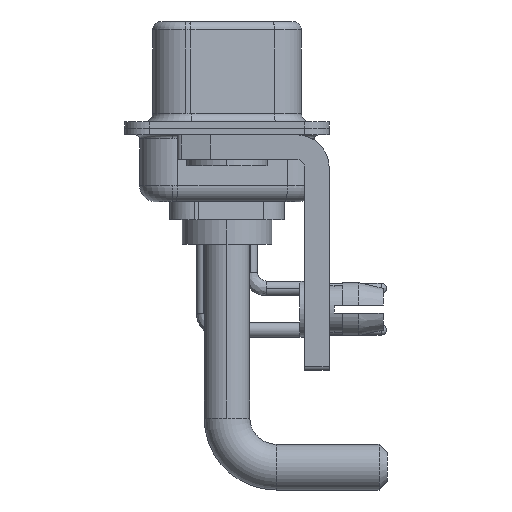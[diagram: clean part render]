
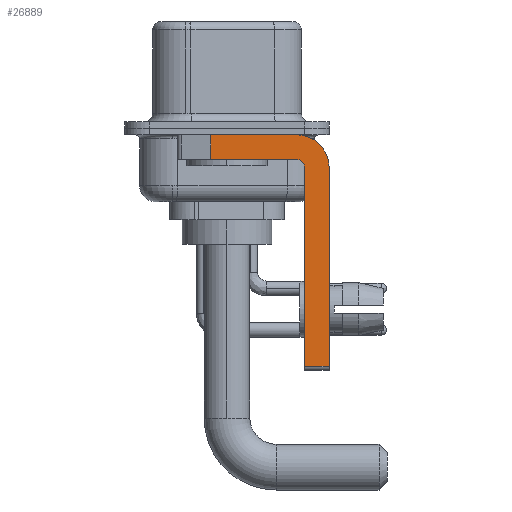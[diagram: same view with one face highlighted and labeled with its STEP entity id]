
A CAD part, left-side view. The second image highlights one B-rep face of the part: STEP entity #26889.
In plain terms, the highlighted planar face has unit normal (-1, 0, 0).
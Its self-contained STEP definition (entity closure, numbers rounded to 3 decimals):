
#29 = VERTEX_POINT ( 'NONE', #8111 ) ;
#87 = DIRECTION ( 'NONE',  ( 0., 0., 1. ) ) ;
#91 = VERTEX_POINT ( 'NONE', #766 ) ;
#352 = VECTOR ( 'NONE', #25271, 1000. ) ;
#766 = CARTESIAN_POINT ( 'NONE',  ( -2.9, 0.978, -1.9 ) ) ;
#917 = VERTEX_POINT ( 'NONE', #10196 ) ;
#934 = EDGE_LOOP ( 'NONE', ( #25266, #8101, #20002, #5341, #11977, #13872, #5453, #2150 ) ) ;
#1042 = EDGE_CURVE ( 'NONE', #917, #29, #13442, .T. ) ;
#2150 = ORIENTED_EDGE ( 'NONE', *, *, #5761, .F. ) ;
#2473 = LINE ( 'NONE', #17156, #7376 ) ;
#2628 = VECTOR ( 'NONE', #23406, 1000. ) ;
#2943 = DIRECTION ( 'NONE',  ( 0., 0., -1. ) ) ;
#3097 = EDGE_CURVE ( 'NONE', #5875, #26290, #18706, .T. ) ;
#3352 = PLANE ( 'NONE',  #24534 ) ;
#3684 = CIRCLE ( 'NONE', #23646, 2. ) ;
#4737 = CARTESIAN_POINT ( 'NONE',  ( -2.9, 0.978, -1.9 ) ) ;
#4861 = CARTESIAN_POINT ( 'NONE',  ( -2.9, -4.25, -1.9 ) ) ;
#4929 = CARTESIAN_POINT ( 'NONE',  ( -2.9, -4.25, -2.4 ) ) ;
#5341 = ORIENTED_EDGE ( 'NONE', *, *, #23295, .F. ) ;
#5453 = ORIENTED_EDGE ( 'NONE', *, *, #11996, .F. ) ;
#5761 = EDGE_CURVE ( 'NONE', #29, #17941, #3684, .T. ) ;
#5875 = VERTEX_POINT ( 'NONE', #6689 ) ;
#5960 = CARTESIAN_POINT ( 'NONE',  ( -2.9, -6.25, -2.4 ) ) ;
#6532 = CARTESIAN_POINT ( 'NONE',  ( -2.9, -4.75, -2.4 ) ) ;
#6689 = CARTESIAN_POINT ( 'NONE',  ( -2.9, -4.75, -14.55 ) ) ;
#6852 = VERTEX_POINT ( 'NONE', #9309 ) ;
#7376 = VECTOR ( 'NONE', #9142, 1000. ) ;
#8101 = ORIENTED_EDGE ( 'NONE', *, *, #12531, .T. ) ;
#8111 = CARTESIAN_POINT ( 'NONE',  ( -2.9, -4.25, -0.4 ) ) ;
#8127 = LINE ( 'NONE', #20635, #11822 ) ;
#8269 = DIRECTION ( 'NONE',  ( 0., 1., 0. ) ) ;
#9142 = DIRECTION ( 'NONE',  ( 0., 0., -1. ) ) ;
#9309 = CARTESIAN_POINT ( 'NONE',  ( -2.9, -6.25, -14.55 ) ) ;
#9338 = CARTESIAN_POINT ( 'NONE',  ( -2.9, -4.25, -2.4 ) ) ;
#9839 = VERTEX_POINT ( 'NONE', #4861 ) ;
#10008 = DIRECTION ( 'NONE',  ( 1., 0., 0. ) ) ;
#10196 = CARTESIAN_POINT ( 'NONE',  ( -2.9, 0.978, -0.4 ) ) ;
#10507 = CARTESIAN_POINT ( 'NONE',  ( -2.9, -4.25, -2.4 ) ) ;
#10664 = DIRECTION ( 'NONE',  ( -1., 0., 0. ) ) ;
#10876 = LINE ( 'NONE', #4737, #23006 ) ;
#11651 = DIRECTION ( 'NONE',  ( 1., 0., 0. ) ) ;
#11822 = VECTOR ( 'NONE', #8269, 1000. ) ;
#11977 = ORIENTED_EDGE ( 'NONE', *, *, #3097, .F. ) ;
#11996 = EDGE_CURVE ( 'NONE', #17941, #6852, #2473, .T. ) ;
#12531 = EDGE_CURVE ( 'NONE', #917, #91, #10876, .T. ) ;
#13248 = DIRECTION ( 'NONE',  ( 0., 0., 1. ) ) ;
#13292 = FACE_OUTER_BOUND ( 'NONE', #934, .T. ) ;
#13442 = LINE ( 'NONE', #21712, #352 ) ;
#13872 = ORIENTED_EDGE ( 'NONE', *, *, #22264, .T. ) ;
#14222 = EDGE_CURVE ( 'NONE', #9839, #91, #8127, .T. ) ;
#14423 = CIRCLE ( 'NONE', #17880, 0.5 ) ;
#15140 = LINE ( 'NONE', #15390, #2628 ) ;
#15390 = CARTESIAN_POINT ( 'NONE',  ( -2.9, -4.25, -14.55 ) ) ;
#15678 = VECTOR ( 'NONE', #87, 1000. ) ;
#16993 = DIRECTION ( 'NONE',  ( 0., 0., -1. ) ) ;
#17156 = CARTESIAN_POINT ( 'NONE',  ( -2.9, -6.25, -2.4 ) ) ;
#17880 = AXIS2_PLACEMENT_3D ( 'NONE', #4929, #10664, #13248 ) ;
#17941 = VERTEX_POINT ( 'NONE', #5960 ) ;
#18706 = LINE ( 'NONE', #24538, #15678 ) ;
#20002 = ORIENTED_EDGE ( 'NONE', *, *, #14222, .F. ) ;
#20635 = CARTESIAN_POINT ( 'NONE',  ( -2.9, -4.25, -1.9 ) ) ;
#21712 = CARTESIAN_POINT ( 'NONE',  ( -2.9, 3., -0.4 ) ) ;
#22264 = EDGE_CURVE ( 'NONE', #5875, #6852, #15140, .T. ) ;
#22347 = DIRECTION ( 'NONE',  ( 0., 0., -1. ) ) ;
#23006 = VECTOR ( 'NONE', #16993, 1000. ) ;
#23295 = EDGE_CURVE ( 'NONE', #26290, #9839, #14423, .T. ) ;
#23406 = DIRECTION ( 'NONE',  ( 0., -1., 0. ) ) ;
#23646 = AXIS2_PLACEMENT_3D ( 'NONE', #10507, #10008, #22347 ) ;
#24534 = AXIS2_PLACEMENT_3D ( 'NONE', #9338, #11651, #2943 ) ;
#24538 = CARTESIAN_POINT ( 'NONE',  ( -2.9, -4.75, -14.8 ) ) ;
#25266 = ORIENTED_EDGE ( 'NONE', *, *, #1042, .F. ) ;
#25271 = DIRECTION ( 'NONE',  ( 0., -1., 0. ) ) ;
#26290 = VERTEX_POINT ( 'NONE', #6532 ) ;
#26889 = ADVANCED_FACE ( 'NONE', ( #13292 ), #3352, .F. ) ;
